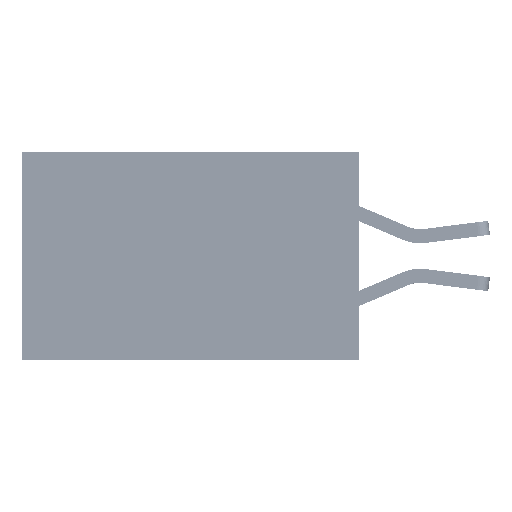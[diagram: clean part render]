
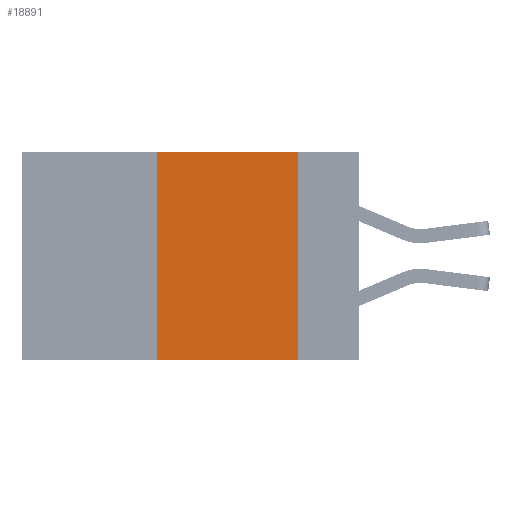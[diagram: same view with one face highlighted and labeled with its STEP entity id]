
A CAD part, left-side view. The second image highlights one B-rep face of the part: STEP entity #18891.
In plain terms, the highlighted planar face has unit normal (-1, 0, 0).
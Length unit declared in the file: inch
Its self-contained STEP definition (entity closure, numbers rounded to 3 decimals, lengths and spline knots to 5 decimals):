
#1935 = EDGE_CURVE ( 'NONE', #21198, #49674, #13072, .T. ) ;
#6591 = DIRECTION ( 'NONE',  ( 0., 0., 1. ) ) ;
#6680 = VECTOR ( 'NONE', #47375, 39.37008 ) ;
#7441 = VECTOR ( 'NONE', #21948, 39.37008 ) ;
#8180 = ORIENTED_EDGE ( 'NONE', *, *, #22411, .F. ) ;
#10044 = CARTESIAN_POINT ( 'NONE',  ( 0., 0.11, 0. ) ) ;
#11157 = CARTESIAN_POINT ( 'NONE',  ( 0., 0.36, -0.37 ) ) ;
#13072 = LINE ( 'NONE', #10044, #7441 ) ;
#13127 = CARTESIAN_POINT ( 'NONE',  ( 0., 0.36, 0. ) ) ;
#16866 = PLANE ( 'NONE',  #50184 ) ;
#18891 = ADVANCED_FACE ( 'NONE', ( #41154 ), #16866, .F. ) ;
#20874 = DIRECTION ( 'NONE',  ( 1., 0., 0. ) ) ;
#21198 = VERTEX_POINT ( 'NONE', #32441 ) ;
#21948 = DIRECTION ( 'NONE',  ( 0., 0., -1. ) ) ;
#22411 = EDGE_CURVE ( 'NONE', #50846, #21198, #24998, .T. ) ;
#22506 = VECTOR ( 'NONE', #40013, 39.37008 ) ;
#22543 = ORIENTED_EDGE ( 'NONE', *, *, #47962, .F. ) ;
#24998 = LINE ( 'NONE', #39313, #22506 ) ;
#29600 = CARTESIAN_POINT ( 'NONE',  ( 0., 0.11, -0.37 ) ) ;
#32441 = CARTESIAN_POINT ( 'NONE',  ( 0., 0.11, 0. ) ) ;
#33139 = EDGE_CURVE ( 'NONE', #40889, #49674, #46592, .T. ) ;
#33394 = DIRECTION ( 'NONE',  ( 0., 0., -1. ) ) ;
#34852 = CARTESIAN_POINT ( 'NONE',  ( 0., 0.36, 0. ) ) ;
#35208 = CARTESIAN_POINT ( 'NONE',  ( 0., 0.6, -0.37 ) ) ;
#39313 = CARTESIAN_POINT ( 'NONE',  ( 0., 0.6, 0. ) ) ;
#40013 = DIRECTION ( 'NONE',  ( 0., -1., 0. ) ) ;
#40433 = ORIENTED_EDGE ( 'NONE', *, *, #33139, .T. ) ;
#40889 = VERTEX_POINT ( 'NONE', #11157 ) ;
#41154 = FACE_OUTER_BOUND ( 'NONE', #42828, .T. ) ;
#42545 = LINE ( 'NONE', #34852, #49406 ) ;
#42828 = EDGE_LOOP ( 'NONE', ( #46124, #8180, #22543, #40433 ) ) ;
#44706 = CARTESIAN_POINT ( 'NONE',  ( 0., 0.6, 0. ) ) ;
#46124 = ORIENTED_EDGE ( 'NONE', *, *, #1935, .F. ) ;
#46592 = LINE ( 'NONE', #35208, #6680 ) ;
#47375 = DIRECTION ( 'NONE',  ( 0., -1., 0. ) ) ;
#47962 = EDGE_CURVE ( 'NONE', #40889, #50846, #42545, .T. ) ;
#49406 = VECTOR ( 'NONE', #6591, 39.37008 ) ;
#49674 = VERTEX_POINT ( 'NONE', #29600 ) ;
#50184 = AXIS2_PLACEMENT_3D ( 'NONE', #44706, #20874, #33394 ) ;
#50846 = VERTEX_POINT ( 'NONE', #13127 ) ;
